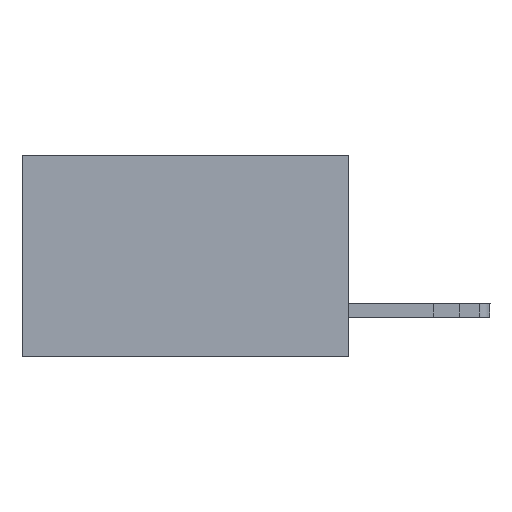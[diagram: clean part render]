
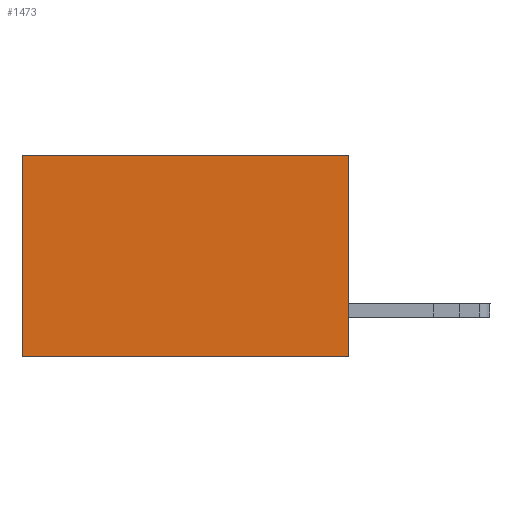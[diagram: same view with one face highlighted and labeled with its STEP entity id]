
A CAD part, left-side view. The second image highlights one B-rep face of the part: STEP entity #1473.
In plain terms, the highlighted planar face has unit normal (-1, 0, 0).
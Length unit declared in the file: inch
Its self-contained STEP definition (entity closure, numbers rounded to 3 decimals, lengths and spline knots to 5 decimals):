
#1196 = LINE ( 'NONE', #18114, #11121 ) ;
#1473 = ADVANCED_FACE ( 'NONE', ( #9418 ), #18547, .F. ) ;
#1629 = LINE ( 'NONE', #1835, #6098 ) ;
#1702 = ORIENTED_EDGE ( 'NONE', *, *, #22666, .T. ) ;
#1798 = EDGE_CURVE ( 'NONE', #7003, #2332, #1196, .T. ) ;
#1835 = CARTESIAN_POINT ( 'NONE',  ( 0.2615, 0., -0.37 ) ) ;
#1972 = CARTESIAN_POINT ( 'NONE',  ( 0.2615, 0., 0. ) ) ;
#2041 = DIRECTION ( 'NONE',  ( 0., 0., -1. ) ) ;
#2332 = VERTEX_POINT ( 'NONE', #22916 ) ;
#3248 = LINE ( 'NONE', #22200, #21648 ) ;
#4704 = CARTESIAN_POINT ( 'NONE',  ( 0.2615, 0.6, 0. ) ) ;
#6098 = VECTOR ( 'NONE', #2041, 39.37008 ) ;
#7003 = VERTEX_POINT ( 'NONE', #4704 ) ;
#7333 = EDGE_LOOP ( 'NONE', ( #9304, #20625, #7836, #1702 ) ) ;
#7836 = ORIENTED_EDGE ( 'NONE', *, *, #8732, .F. ) ;
#8732 = EDGE_CURVE ( 'NONE', #17297, #9890, #1629, .T. ) ;
#9304 = ORIENTED_EDGE ( 'NONE', *, *, #1798, .T. ) ;
#9418 = FACE_OUTER_BOUND ( 'NONE', #7333, .T. ) ;
#9890 = VERTEX_POINT ( 'NONE', #16227 ) ;
#11121 = VECTOR ( 'NONE', #18054, 39.37008 ) ;
#12072 = VECTOR ( 'NONE', #14940, 39.37008 ) ;
#12581 = CARTESIAN_POINT ( 'NONE',  ( 0.2615, 0., 0. ) ) ;
#13274 = AXIS2_PLACEMENT_3D ( 'NONE', #17607, #17603, #16853 ) ;
#13753 = LINE ( 'NONE', #1972, #12072 ) ;
#13802 = DIRECTION ( 'NONE',  ( 0., 1., 0. ) ) ;
#14940 = DIRECTION ( 'NONE',  ( 0., 1., 0. ) ) ;
#16227 = CARTESIAN_POINT ( 'NONE',  ( 0.2615, 0., -0.37 ) ) ;
#16853 = DIRECTION ( 'NONE',  ( 0., 0., -1. ) ) ;
#17297 = VERTEX_POINT ( 'NONE', #12581 ) ;
#17603 = DIRECTION ( 'NONE',  ( 1., 0., 0. ) ) ;
#17607 = CARTESIAN_POINT ( 'NONE',  ( 0.2615, 0., -0.37 ) ) ;
#18054 = DIRECTION ( 'NONE',  ( 0., 0., -1. ) ) ;
#18114 = CARTESIAN_POINT ( 'NONE',  ( 0.2615, 0.6, -0.37 ) ) ;
#18547 = PLANE ( 'NONE',  #13274 ) ;
#18613 = EDGE_CURVE ( 'NONE', #9890, #2332, #3248, .T. ) ;
#20625 = ORIENTED_EDGE ( 'NONE', *, *, #18613, .F. ) ;
#21648 = VECTOR ( 'NONE', #13802, 39.37008 ) ;
#22200 = CARTESIAN_POINT ( 'NONE',  ( 0.2615, 0., -0.37 ) ) ;
#22666 = EDGE_CURVE ( 'NONE', #17297, #7003, #13753, .T. ) ;
#22916 = CARTESIAN_POINT ( 'NONE',  ( 0.2615, 0.6, -0.37 ) ) ;
